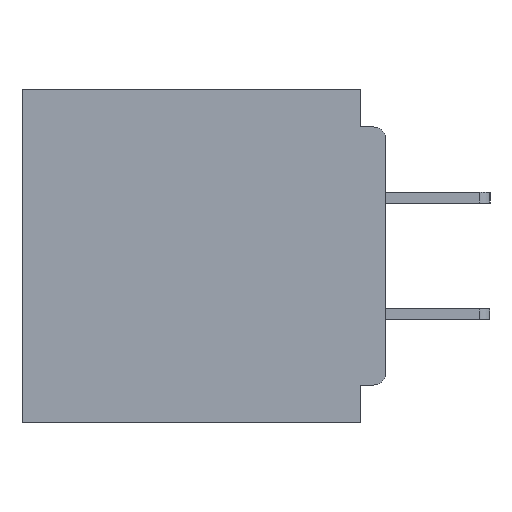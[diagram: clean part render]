
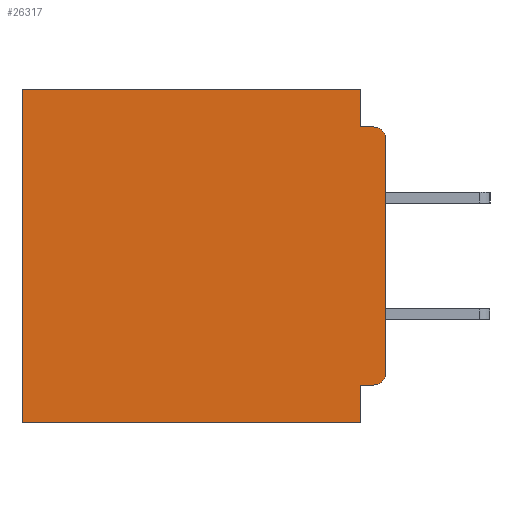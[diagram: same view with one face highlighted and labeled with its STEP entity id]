
A CAD part, left-side view. The second image highlights one B-rep face of the part: STEP entity #26317.
In plain terms, the highlighted planar face has unit normal (-1, 0, 0).
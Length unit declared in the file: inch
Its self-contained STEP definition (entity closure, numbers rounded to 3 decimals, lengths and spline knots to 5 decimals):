
#1 = DIRECTION ( 'NONE',  ( -1., 0., 0. ) ) ;
#65 = DIRECTION ( 'NONE',  ( 0., 0., -1. ) ) ;
#383 = EDGE_CURVE ( 'NONE', #40779, #1866, #36203, .T. ) ;
#1371 = DIRECTION ( 'NONE',  ( 0., 0., -1. ) ) ;
#1378 = EDGE_CURVE ( 'NONE', #35061, #36430, #29920, .T. ) ;
#1581 = DIRECTION ( 'NONE',  ( 0., 1., 0. ) ) ;
#1866 = VERTEX_POINT ( 'NONE', #32149 ) ;
#1868 = EDGE_CURVE ( 'NONE', #14079, #21610, #18025, .T. ) ;
#3512 = ORIENTED_EDGE ( 'NONE', *, *, #16673, .T. ) ;
#3768 = CARTESIAN_POINT ( 'NONE',  ( 0.3, 0.031, -0.4 ) ) ;
#4160 = CARTESIAN_POINT ( 'NONE',  ( 0.3, 0.015, -0.355 ) ) ;
#4273 = CARTESIAN_POINT ( 'NONE',  ( 0.3, 0.015, -0.045 ) ) ;
#5001 = CARTESIAN_POINT ( 'NONE',  ( 0.3, 0., -0.4 ) ) ;
#5010 = AXIS2_PLACEMENT_3D ( 'NONE', #29717, #9864, #33026 ) ;
#5410 = CARTESIAN_POINT ( 'NONE',  ( 0.3, 0., -0.4 ) ) ;
#8095 = CARTESIAN_POINT ( 'NONE',  ( 0.3, 0.437, 0. ) ) ;
#8408 = DIRECTION ( 'NONE',  ( 1., 0., 0. ) ) ;
#8780 = ORIENTED_EDGE ( 'NONE', *, *, #1868, .T. ) ;
#9800 = VECTOR ( 'NONE', #1581, 39.37008 ) ;
#9864 = DIRECTION ( 'NONE',  ( -1., 0., 0. ) ) ;
#10118 = ORIENTED_EDGE ( 'NONE', *, *, #19500, .F. ) ;
#10179 = VECTOR ( 'NONE', #32046, 39.37008 ) ;
#10581 = EDGE_CURVE ( 'NONE', #21610, #14799, #18823, .T. ) ;
#11180 = LINE ( 'NONE', #28101, #35492 ) ;
#11457 = LINE ( 'NONE', #23413, #29048 ) ;
#11684 = ORIENTED_EDGE ( 'NONE', *, *, #34304, .F. ) ;
#12407 = DIRECTION ( 'NONE',  ( 0., -1., 0. ) ) ;
#12456 = AXIS2_PLACEMENT_3D ( 'NONE', #5001, #8408, #31601 ) ;
#12527 = VECTOR ( 'NONE', #1371, 39.37008 ) ;
#12769 = CARTESIAN_POINT ( 'NONE',  ( 0.3, 0.031, 0. ) ) ;
#14079 = VERTEX_POINT ( 'NONE', #12769 ) ;
#14383 = CIRCLE ( 'NONE', #25003, 0.015 ) ;
#14529 = ORIENTED_EDGE ( 'NONE', *, *, #17647, .F. ) ;
#14799 = VERTEX_POINT ( 'NONE', #19845 ) ;
#16673 = EDGE_CURVE ( 'NONE', #40779, #19862, #14383, .T. ) ;
#17149 = CARTESIAN_POINT ( 'NONE',  ( 0.3, 0.437, -0.4 ) ) ;
#17174 = ORIENTED_EDGE ( 'NONE', *, *, #30654, .F. ) ;
#17647 = EDGE_CURVE ( 'NONE', #41965, #14799, #25696, .T. ) ;
#18025 = LINE ( 'NONE', #34786, #10179 ) ;
#18823 = LINE ( 'NONE', #17149, #35347 ) ;
#19500 = EDGE_CURVE ( 'NONE', #14079, #35061, #41041, .T. ) ;
#19845 = CARTESIAN_POINT ( 'NONE',  ( 0.3, 0.437, -0.4 ) ) ;
#19862 = VERTEX_POINT ( 'NONE', #38636 ) ;
#19991 = CARTESIAN_POINT ( 'NONE',  ( 0.3, 0.015, -0.34 ) ) ;
#20457 = DIRECTION ( 'NONE',  ( 0., 0., -1. ) ) ;
#21237 = EDGE_CURVE ( 'NONE', #41933, #36430, #24803, .T. ) ;
#21610 = VERTEX_POINT ( 'NONE', #8095 ) ;
#23337 = DIRECTION ( 'NONE',  ( 0., 0., -1. ) ) ;
#23413 = CARTESIAN_POINT ( 'NONE',  ( 0.3, 0., -0.4 ) ) ;
#23941 = CARTESIAN_POINT ( 'NONE',  ( 0.3, 0.031, -0.045 ) ) ;
#24803 = CIRCLE ( 'NONE', #5010, 0.015 ) ;
#24975 = PLANE ( 'NONE',  #12456 ) ;
#25003 = AXIS2_PLACEMENT_3D ( 'NONE', #19991, #1, #23337 ) ;
#25696 = LINE ( 'NONE', #5410, #42225 ) ;
#25878 = FACE_OUTER_BOUND ( 'NONE', #29383, .T. ) ;
#26317 = ADVANCED_FACE ( 'NONE', ( #25878 ), #24975, .F. ) ;
#28101 = CARTESIAN_POINT ( 'NONE',  ( 0.3, 0.031, -0.4 ) ) ;
#29048 = VECTOR ( 'NONE', #65, 39.37008 ) ;
#29383 = EDGE_LOOP ( 'NONE', ( #11684, #40122, #30152, #10118, #8780, #40927, #14529, #17174, #42473, #3512 ) ) ;
#29717 = CARTESIAN_POINT ( 'NONE',  ( 0.3, 0.015, -0.06 ) ) ;
#29920 = LINE ( 'NONE', #40219, #39756 ) ;
#30152 = ORIENTED_EDGE ( 'NONE', *, *, #1378, .F. ) ;
#30654 = EDGE_CURVE ( 'NONE', #1866, #41965, #11180, .T. ) ;
#31430 = DIRECTION ( 'NONE',  ( 0., 0., -1. ) ) ;
#31601 = DIRECTION ( 'NONE',  ( 0., 0., -1. ) ) ;
#32046 = DIRECTION ( 'NONE',  ( 0., 1., 0. ) ) ;
#32149 = CARTESIAN_POINT ( 'NONE',  ( 0.3, 0.031, -0.355 ) ) ;
#33026 = DIRECTION ( 'NONE',  ( 0., 0., -1. ) ) ;
#33539 = CARTESIAN_POINT ( 'NONE',  ( 0.3, 0., -0.06 ) ) ;
#34304 = EDGE_CURVE ( 'NONE', #41933, #19862, #11457, .T. ) ;
#34478 = CARTESIAN_POINT ( 'NONE',  ( 0.3, 0.031, 0. ) ) ;
#34786 = CARTESIAN_POINT ( 'NONE',  ( 0.3, 0., 0. ) ) ;
#35061 = VERTEX_POINT ( 'NONE', #23941 ) ;
#35332 = DIRECTION ( 'NONE',  ( 0., 1., 0. ) ) ;
#35347 = VECTOR ( 'NONE', #20457, 39.37008 ) ;
#35492 = VECTOR ( 'NONE', #31430, 39.37008 ) ;
#36203 = LINE ( 'NONE', #42203, #9800 ) ;
#36430 = VERTEX_POINT ( 'NONE', #4273 ) ;
#38636 = CARTESIAN_POINT ( 'NONE',  ( 0.3, 0., -0.34 ) ) ;
#39756 = VECTOR ( 'NONE', #12407, 39.37008 ) ;
#40122 = ORIENTED_EDGE ( 'NONE', *, *, #21237, .T. ) ;
#40219 = CARTESIAN_POINT ( 'NONE',  ( 0.3, 0., -0.045 ) ) ;
#40779 = VERTEX_POINT ( 'NONE', #4160 ) ;
#40927 = ORIENTED_EDGE ( 'NONE', *, *, #10581, .T. ) ;
#41041 = LINE ( 'NONE', #34478, #12527 ) ;
#41933 = VERTEX_POINT ( 'NONE', #33539 ) ;
#41965 = VERTEX_POINT ( 'NONE', #3768 ) ;
#42203 = CARTESIAN_POINT ( 'NONE',  ( 0.3, 0., -0.355 ) ) ;
#42225 = VECTOR ( 'NONE', #35332, 39.37008 ) ;
#42473 = ORIENTED_EDGE ( 'NONE', *, *, #383, .F. ) ;
